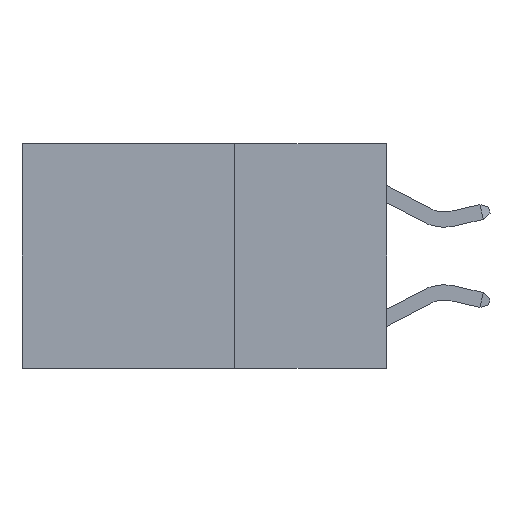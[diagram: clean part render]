
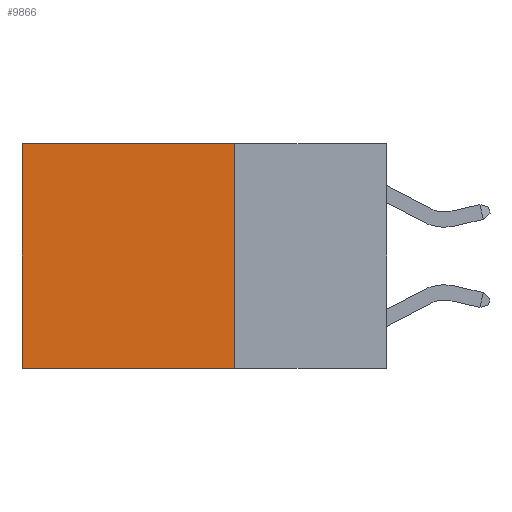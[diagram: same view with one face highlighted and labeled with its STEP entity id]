
A CAD part, left-side view. The second image highlights one B-rep face of the part: STEP entity #9866.
In plain terms, the highlighted planar face has unit normal (-1, 0, 0).
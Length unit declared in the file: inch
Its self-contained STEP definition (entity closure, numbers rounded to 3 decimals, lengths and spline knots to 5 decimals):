
#7 = ORIENTED_EDGE ( 'NONE', *, *, #4843, .T. ) ;
#853 = EDGE_CURVE ( 'NONE', #2184, #5390, #8768, .T. ) ;
#1249 = VERTEX_POINT ( 'NONE', #6759 ) ;
#1540 = ORIENTED_EDGE ( 'NONE', *, *, #9685, .F. ) ;
#1580 = LINE ( 'NONE', #9118, #8004 ) ;
#2151 = LINE ( 'NONE', #4942, #6396 ) ;
#2156 = DIRECTION ( 'NONE',  ( 1., 0., 0. ) ) ;
#2184 = VERTEX_POINT ( 'NONE', #9461 ) ;
#2515 = DIRECTION ( 'NONE',  ( 0., 1., 0. ) ) ;
#2994 = DIRECTION ( 'NONE',  ( 0., 1., 0. ) ) ;
#3810 = PLANE ( 'NONE',  #4497 ) ;
#3976 = FACE_OUTER_BOUND ( 'NONE', #10077, .T. ) ;
#4497 = AXIS2_PLACEMENT_3D ( 'NONE', #10582, #2156, #8021 ) ;
#4547 = VERTEX_POINT ( 'NONE', #7857 ) ;
#4843 = EDGE_CURVE ( 'NONE', #1249, #2184, #1580, .T. ) ;
#4942 = CARTESIAN_POINT ( 'NONE',  ( 0.2625, 0.25, 0. ) ) ;
#5390 = VERTEX_POINT ( 'NONE', #9895 ) ;
#5507 = CARTESIAN_POINT ( 'NONE',  ( 0.2625, 0.25, -0.37 ) ) ;
#5918 = LINE ( 'NONE', #5507, #10109 ) ;
#6349 = VECTOR ( 'NONE', #9285, 39.37008 ) ;
#6396 = VECTOR ( 'NONE', #9065, 39.37008 ) ;
#6474 = ORIENTED_EDGE ( 'NONE', *, *, #7071, .F. ) ;
#6759 = CARTESIAN_POINT ( 'NONE',  ( 0.2625, 0.25, 0. ) ) ;
#6827 = CARTESIAN_POINT ( 'NONE',  ( 0.2625, 0.6, 0. ) ) ;
#7071 = EDGE_CURVE ( 'NONE', #4547, #5390, #5918, .T. ) ;
#7857 = CARTESIAN_POINT ( 'NONE',  ( 0.2625, 0.25, -0.37 ) ) ;
#8004 = VECTOR ( 'NONE', #2515, 39.37008 ) ;
#8021 = DIRECTION ( 'NONE',  ( 0., 0., -1. ) ) ;
#8768 = LINE ( 'NONE', #6827, #6349 ) ;
#9065 = DIRECTION ( 'NONE',  ( 0., 0., -1. ) ) ;
#9118 = CARTESIAN_POINT ( 'NONE',  ( 0.2625, 0.25, 0. ) ) ;
#9285 = DIRECTION ( 'NONE',  ( 0., 0., -1. ) ) ;
#9461 = CARTESIAN_POINT ( 'NONE',  ( 0.2625, 0.6, 0. ) ) ;
#9685 = EDGE_CURVE ( 'NONE', #1249, #4547, #2151, .T. ) ;
#9835 = ORIENTED_EDGE ( 'NONE', *, *, #853, .T. ) ;
#9866 = ADVANCED_FACE ( 'NONE', ( #3976 ), #3810, .F. ) ;
#9895 = CARTESIAN_POINT ( 'NONE',  ( 0.2625, 0.6, -0.37 ) ) ;
#10077 = EDGE_LOOP ( 'NONE', ( #9835, #6474, #1540, #7 ) ) ;
#10109 = VECTOR ( 'NONE', #2994, 39.37008 ) ;
#10582 = CARTESIAN_POINT ( 'NONE',  ( 0.2625, 0.25, 0. ) ) ;
